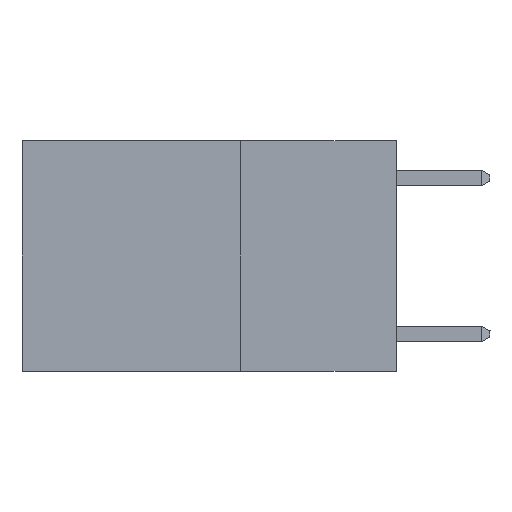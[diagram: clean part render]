
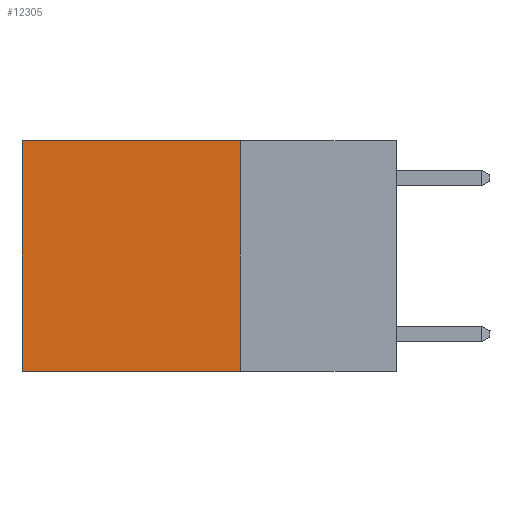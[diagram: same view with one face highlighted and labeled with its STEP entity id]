
A CAD part, left-side view. The second image highlights one B-rep face of the part: STEP entity #12305.
In plain terms, the highlighted planar face has unit normal (-1, 0, 0).
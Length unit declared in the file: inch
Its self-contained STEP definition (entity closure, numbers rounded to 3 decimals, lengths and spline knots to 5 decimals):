
#1221 = LINE ( 'NONE', #18752, #1390 ) ;
#1390 = VECTOR ( 'NONE', #4090, 39.37008 ) ;
#2132 = DIRECTION ( 'NONE',  ( 0., 0., -1. ) ) ;
#4086 = CARTESIAN_POINT ( 'NONE',  ( 0.2625, 0.25, 0. ) ) ;
#4090 = DIRECTION ( 'NONE',  ( 0., 0., -1. ) ) ;
#4179 = EDGE_CURVE ( 'NONE', #16287, #13520, #6895, .T. ) ;
#4832 = EDGE_CURVE ( 'NONE', #28214, #16287, #1221, .T. ) ;
#5001 = EDGE_LOOP ( 'NONE', ( #15757, #8626, #6785, #24776 ) ) ;
#5042 = VECTOR ( 'NONE', #26015, 39.37008 ) ;
#6155 = CARTESIAN_POINT ( 'NONE',  ( 0.2625, 0.25, -0.37 ) ) ;
#6529 = DIRECTION ( 'NONE',  ( 0., 0., -1. ) ) ;
#6785 = ORIENTED_EDGE ( 'NONE', *, *, #4832, .F. ) ;
#6836 = VECTOR ( 'NONE', #21224, 39.37008 ) ;
#6895 = LINE ( 'NONE', #30557, #6836 ) ;
#8448 = LINE ( 'NONE', #28642, #14929 ) ;
#8626 = ORIENTED_EDGE ( 'NONE', *, *, #4179, .F. ) ;
#9155 = FACE_OUTER_BOUND ( 'NONE', #5001, .T. ) ;
#9639 = CARTESIAN_POINT ( 'NONE',  ( 0.2625, 0.25, 0. ) ) ;
#11243 = PLANE ( 'NONE',  #22256 ) ;
#11672 = CARTESIAN_POINT ( 'NONE',  ( 0.2625, 0.25, 0. ) ) ;
#11846 = CARTESIAN_POINT ( 'NONE',  ( 0.2625, 0.6, 0. ) ) ;
#12305 = ADVANCED_FACE ( 'NONE', ( #9155 ), #11243, .F. ) ;
#12306 = LINE ( 'NONE', #11672, #5042 ) ;
#13520 = VERTEX_POINT ( 'NONE', #22755 ) ;
#14929 = VECTOR ( 'NONE', #2132, 39.37008 ) ;
#15757 = ORIENTED_EDGE ( 'NONE', *, *, #26843, .T. ) ;
#16287 = VERTEX_POINT ( 'NONE', #6155 ) ;
#18752 = CARTESIAN_POINT ( 'NONE',  ( 0.2625, 0.25, 0. ) ) ;
#21121 = DIRECTION ( 'NONE',  ( 1., 0., 0. ) ) ;
#21224 = DIRECTION ( 'NONE',  ( 0., 1., 0. ) ) ;
#22256 = AXIS2_PLACEMENT_3D ( 'NONE', #4086, #21121, #6529 ) ;
#22755 = CARTESIAN_POINT ( 'NONE',  ( 0.2625, 0.6, -0.37 ) ) ;
#24776 = ORIENTED_EDGE ( 'NONE', *, *, #26252, .T. ) ;
#26015 = DIRECTION ( 'NONE',  ( 0., 1., 0. ) ) ;
#26252 = EDGE_CURVE ( 'NONE', #28214, #26817, #12306, .T. ) ;
#26817 = VERTEX_POINT ( 'NONE', #11846 ) ;
#26843 = EDGE_CURVE ( 'NONE', #26817, #13520, #8448, .T. ) ;
#28214 = VERTEX_POINT ( 'NONE', #9639 ) ;
#28642 = CARTESIAN_POINT ( 'NONE',  ( 0.2625, 0.6, 0. ) ) ;
#30557 = CARTESIAN_POINT ( 'NONE',  ( 0.2625, 0.25, -0.37 ) ) ;
